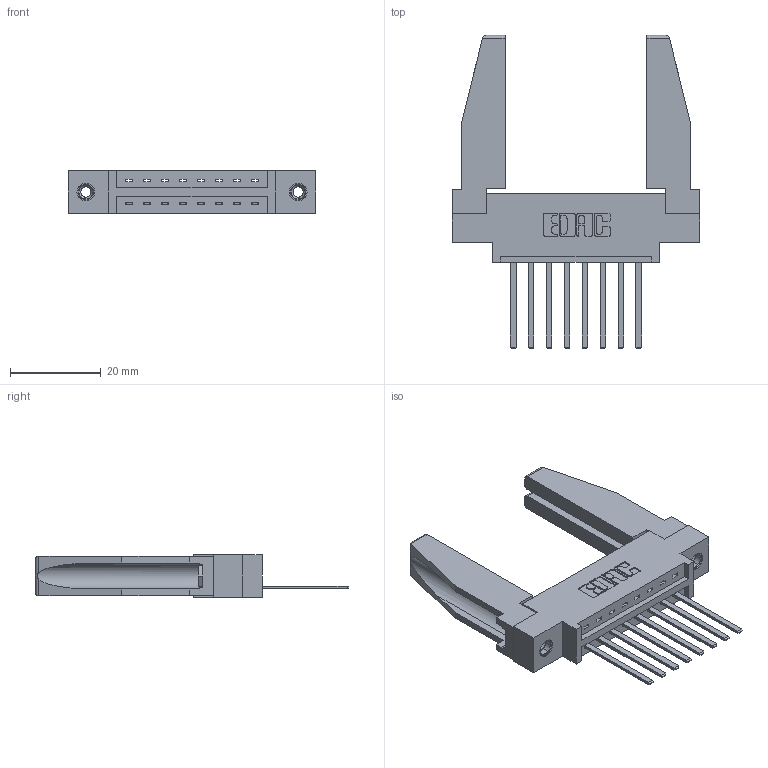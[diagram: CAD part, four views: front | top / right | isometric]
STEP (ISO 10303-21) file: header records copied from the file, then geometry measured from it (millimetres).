
FILE_DESCRIPTION (( 'STEP AP203' ), '1' );
FILE_NAME ('387-008-544-678.STEP', '2019-10-02T04:16:02', ( '' ), ( '' ), 'SwSTEP 2.0', 'SolidWorks 2016', '' );
FILE_SCHEMA (( 'CONFIG_CONTROL_DESIGN' ));
Length unit declared in the file: inch
Products named in the file (5): 345-292-001_345-293-144; 337 Part_0.170 Offset - 0.156 Dia-TI; 307-220-078; 345-250-001_345-250-001-102; 387-008-544-678
Assembly tree (13 placements, depth 2):
  387-008-544-678
    337 Part_0.170 Offset - 0.156 Dia-TI
    345-292-001_345-293-144  x8
    345-250-001_345-250-001-102  x2
    307-220-078  x2
Bounding box: 54.71 x 69.09 x 9.4 mm (x, y, z)
Volume: 9229.4 mm3; surface area: 9460 mm2
Topology: 13 solids, 13 shells, 696 faces, 2013 edges, 1322 vertices
Faces by surface type: plane 494, cylinder 186, cone 12, torus 4
Entity records: 12732 total; most frequent: CARTESIAN_POINT 2208, ORIENTED_EDGE 2108, DIRECTION 1934, EDGE_CURVE 1054, VECTOR 892, LINE 892, VERTEX_POINT 696, AXIS2_PLACEMENT_3D 521
